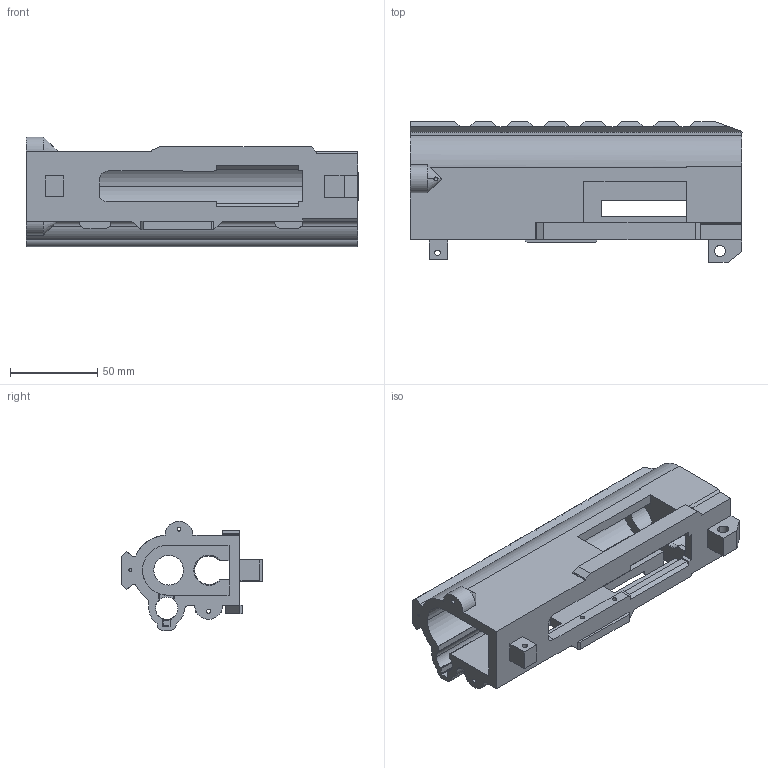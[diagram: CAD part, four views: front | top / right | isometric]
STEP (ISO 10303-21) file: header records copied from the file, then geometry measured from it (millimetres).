
FILE_DESCRIPTION(('STEP AP214'),'1');
FILE_NAME('WTF9MVE Upper Receiver.stp','2020-09-01T22:10:43',(' '),(' '),'Spatial InterOp 3D',' ',' ');
FILE_SCHEMA(('AUTOMOTIVE_DESIGN { 1 0 10303 214 1 1 1 1 }'));
Length unit declared in the file: metre
Products named in the file (1): Solid
Bounding box: 190.38 x 80.5 x 62.82 mm (x, y, z)
Volume: 220783.9 mm3; surface area: 81424.8 mm2
Topology: 1 solids, 1 shells, 267 faces, 747 edges, 479 vertices
Faces by surface type: plane 152, cylinder 84, cone 16, torus 9, sphere 4, bspline 2
Entity records: 8983 total; most frequent: CARTESIAN_POINT 1944, ORIENTED_EDGE 1490, DIRECTION 1454, EDGE_CURVE 745, LINE 508, VECTOR 508, VERTEX_POINT 479, AXIS2_PLACEMENT_3D 473
